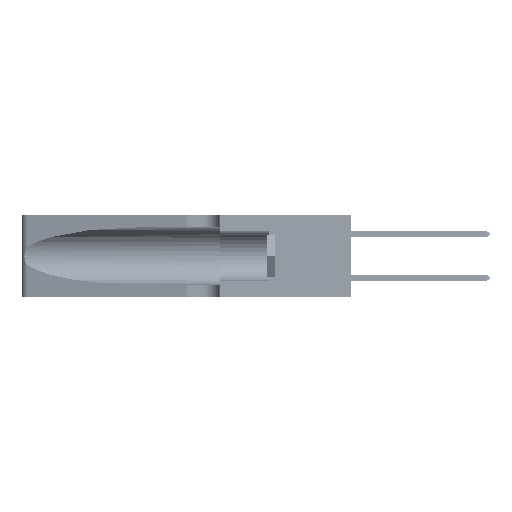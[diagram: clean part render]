
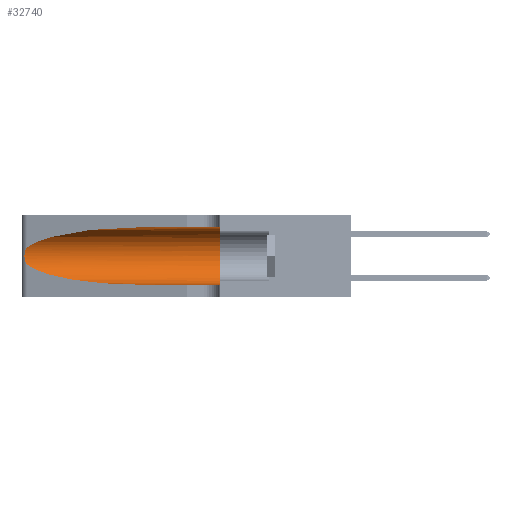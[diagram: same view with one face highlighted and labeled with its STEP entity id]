
A CAD part, left-side view. The second image highlights one B-rep face of the part: STEP entity #32740.
In plain terms, the highlighted cylindrical face has radius 3.308 mm (diameter 6.617 mm), a partial arc.
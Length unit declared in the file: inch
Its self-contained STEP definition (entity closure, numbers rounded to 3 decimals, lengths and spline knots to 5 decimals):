
#272 = DIRECTION ( 'NONE',  ( 0., -1., 0. ) ) ;
#298 = CARTESIAN_POINT ( 'NONE',  ( 0.25487, 1.22718, 0.22369 ) ) ;
#468 = CARTESIAN_POINT ( 'NONE',  ( 0.25487, 1.22718, 0.14631 ) ) ;
#616 =( BOUNDED_CURVE ( )  B_SPLINE_CURVE ( 3, ( #5601, #9537, #37026, #13533 ),
 .UNSPECIFIED., .F., .T. ) 
 B_SPLINE_CURVE_WITH_KNOTS ( ( 4, 4 ),
 ( 3.44316, 4.71239 ),
 .UNSPECIFIED. ) 
 CURVE ( )  GEOMETRIC_REPRESENTATION_ITEM ( )  RATIONAL_B_SPLINE_CURVE ( ( 1., 0.87, 0.87, 1. ) ) 
 REPRESENTATION_ITEM ( '' )  );
#2106 = AXIS2_PLACEMENT_3D ( 'NONE', #47146, #272, #20013 ) ;
#2373 = FACE_OUTER_BOUND ( 'NONE', #19684, .T. ) ;
#3607 = VERTEX_POINT ( 'NONE', #34609 ) ;
#4311 = CARTESIAN_POINT ( 'NONE',  ( 0.25639, 1.23184, 0.21858 ) ) ;
#5601 = CARTESIAN_POINT ( 'NONE',  ( 0.25487, 1.22718, 0.14631 ) ) ;
#5656 = CARTESIAN_POINT ( 'NONE',  ( 0.1305, 0.35, 0.31525 ) ) ;
#6435 = CARTESIAN_POINT ( 'NONE',  ( 0.2373, 1.15595, 0.28018 ) ) ;
#8283 = CARTESIAN_POINT ( 'NONE',  ( 0.25854, 1.2359, 0.20912 ) ) ;
#9462 = EDGE_CURVE ( 'NONE', #39287, #25666, #23496, .T. ) ;
#9537 = CARTESIAN_POINT ( 'NONE',  ( 0.2373, 1.15595, 0.08982 ) ) ;
#9792 = B_SPLINE_CURVE_WITH_KNOTS ( 'NONE', 3,
 ( #298, #27896, #4311, #31812, #8283, #35735, #12245, #39661, #16237, #43599, #20210, #47504, #24128, #468 ),
 .UNSPECIFIED., .F., .F.,
 ( 4, 2, 2, 2, 2, 2, 4 ),
 ( 0., 0.00027, 0.00053, 0.00107, 0.0016, 0.00187, 0.00214 ),
 .UNSPECIFIED. ) ;
#9807 = CARTESIAN_POINT ( 'NONE',  ( 0.25487, 1.22718, 0.22369 ) ) ;
#10451 = VERTEX_POINT ( 'NONE', #36939 ) ;
#12245 = CARTESIAN_POINT ( 'NONE',  ( 0.26075, 1.23896, 0.19203 ) ) ;
#13533 = CARTESIAN_POINT ( 'NONE',  ( 0.1305, 0.72297, 0.05475 ) ) ;
#14155 = CARTESIAN_POINT ( 'NONE',  ( 0.1305, 0.35, 0.185 ) ) ;
#16237 = CARTESIAN_POINT ( 'NONE',  ( 0.26017, 1.23833, 0.17102 ) ) ;
#16681 = AXIS2_PLACEMENT_3D ( 'NONE', #14155, #41552, #18159 ) ;
#17042 = VECTOR ( 'NONE', #27331, 39.37008 ) ;
#17701 = EDGE_CURVE ( 'NONE', #22177, #10451, #9792, .T. ) ;
#18159 = DIRECTION ( 'NONE',  ( 0., 0., 1. ) ) ;
#18641 = EDGE_CURVE ( 'NONE', #10451, #39287, #616, .T. ) ;
#19410 = EDGE_CURVE ( 'NONE', #43944, #25666, #30850, .T. ) ;
#19684 = EDGE_LOOP ( 'NONE', ( #49381, #46248, #47653, #27800, #36561, #49912 ) ) ;
#19989 = CARTESIAN_POINT ( 'NONE',  ( 0.1305, 1.61858, 0.05475 ) ) ;
#20013 = DIRECTION ( 'NONE',  ( 0., 0., -1. ) ) ;
#20210 = CARTESIAN_POINT ( 'NONE',  ( 0.25789, 1.23486, 0.15765 ) ) ;
#22105 = CYLINDRICAL_SURFACE ( 'NONE', #2106, 0.13025 ) ;
#22177 = VERTEX_POINT ( 'NONE', #9807 ) ;
#23496 = LINE ( 'NONE', #19989, #49690 ) ;
#24128 = CARTESIAN_POINT ( 'NONE',  ( 0.25555, 1.22993, 0.14849 ) ) ;
#24944 = EDGE_CURVE ( 'NONE', #3607, #22177, #33433, .T. ) ;
#25666 = VERTEX_POINT ( 'NONE', #37952 ) ;
#27168 = CARTESIAN_POINT ( 'NONE',  ( 0.1305, 1.61858, 0.31525 ) ) ;
#27331 = DIRECTION ( 'NONE',  ( 0., -1., 0. ) ) ;
#27433 = LINE ( 'NONE', #27168, #17042 ) ;
#27800 = ORIENTED_EDGE ( 'NONE', *, *, #9462, .T. ) ;
#27896 = CARTESIAN_POINT ( 'NONE',  ( 0.25555, 1.22994, 0.2215 ) ) ;
#30850 = CIRCLE ( 'NONE', #16681, 0.13025 ) ;
#31812 = CARTESIAN_POINT ( 'NONE',  ( 0.25787, 1.23484, 0.2124 ) ) ;
#32740 = ADVANCED_FACE ( 'NONE', ( #2373 ), #22105, .F. ) ;
#33433 =( BOUNDED_CURVE ( )  B_SPLINE_CURVE ( 3, ( #33778, #49402, #6435, #33943 ),
 .UNSPECIFIED., .F., .T. ) 
 B_SPLINE_CURVE_WITH_KNOTS ( ( 4, 4 ),
 ( 1.5708, 2.84003 ),
 .UNSPECIFIED. ) 
 CURVE ( )  GEOMETRIC_REPRESENTATION_ITEM ( )  RATIONAL_B_SPLINE_CURVE ( ( 1., 0.87, 0.87, 1. ) ) 
 REPRESENTATION_ITEM ( '' )  );
#33778 = CARTESIAN_POINT ( 'NONE',  ( 0.1305, 0.72297, 0.31525 ) ) ;
#33943 = CARTESIAN_POINT ( 'NONE',  ( 0.25487, 1.22718, 0.22369 ) ) ;
#34609 = CARTESIAN_POINT ( 'NONE',  ( 0.1305, 0.72297, 0.31525 ) ) ;
#35735 = CARTESIAN_POINT ( 'NONE',  ( 0.26018, 1.23835, 0.19895 ) ) ;
#36561 = ORIENTED_EDGE ( 'NONE', *, *, #19410, .F. ) ;
#36939 = CARTESIAN_POINT ( 'NONE',  ( 0.25487, 1.22718, 0.14631 ) ) ;
#37026 = CARTESIAN_POINT ( 'NONE',  ( 0.18966, 0.96281, 0.05475 ) ) ;
#37302 = CARTESIAN_POINT ( 'NONE',  ( 0.1305, 0.72297, 0.05475 ) ) ;
#37952 = CARTESIAN_POINT ( 'NONE',  ( 0.1305, 0.35, 0.05475 ) ) ;
#39287 = VERTEX_POINT ( 'NONE', #37302 ) ;
#39452 = DIRECTION ( 'NONE',  ( 0., -1., 0. ) ) ;
#39661 = CARTESIAN_POINT ( 'NONE',  ( 0.26075, 1.23896, 0.178 ) ) ;
#41552 = DIRECTION ( 'NONE',  ( 0., 1., 0. ) ) ;
#43599 = CARTESIAN_POINT ( 'NONE',  ( 0.25856, 1.23593, 0.16098 ) ) ;
#43944 = VERTEX_POINT ( 'NONE', #5656 ) ;
#46248 = ORIENTED_EDGE ( 'NONE', *, *, #17701, .T. ) ;
#47146 = CARTESIAN_POINT ( 'NONE',  ( 0.1305, 1.61858, 0.185 ) ) ;
#47504 = CARTESIAN_POINT ( 'NONE',  ( 0.25639, 1.23186, 0.15144 ) ) ;
#47653 = ORIENTED_EDGE ( 'NONE', *, *, #18641, .T. ) ;
#49381 = ORIENTED_EDGE ( 'NONE', *, *, #24944, .T. ) ;
#49402 = CARTESIAN_POINT ( 'NONE',  ( 0.18966, 0.96281, 0.31525 ) ) ;
#49576 = EDGE_CURVE ( 'NONE', #3607, #43944, #27433, .T. ) ;
#49690 = VECTOR ( 'NONE', #39452, 39.37008 ) ;
#49912 = ORIENTED_EDGE ( 'NONE', *, *, #49576, .F. ) ;
